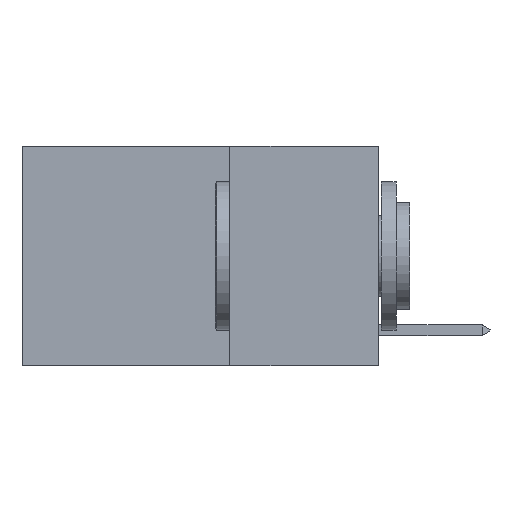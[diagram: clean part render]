
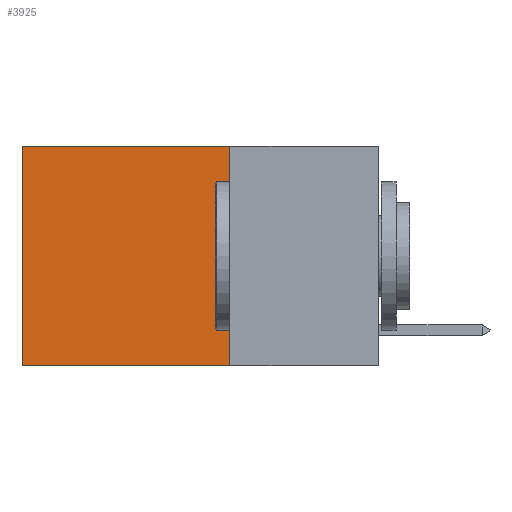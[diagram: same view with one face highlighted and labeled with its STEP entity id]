
A CAD part, left-side view. The second image highlights one B-rep face of the part: STEP entity #3925.
In plain terms, the highlighted planar face has unit normal (-1, 0, 0).
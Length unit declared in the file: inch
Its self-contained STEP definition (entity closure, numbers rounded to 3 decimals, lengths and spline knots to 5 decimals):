
#466 = CARTESIAN_POINT ( 'NONE',  ( 0.2625, 0.6, -0.37 ) ) ;
#601 = CARTESIAN_POINT ( 'NONE',  ( 0.2625, 0.25, 0. ) ) ;
#702 = DIRECTION ( 'NONE',  ( 0., 0., -1. ) ) ;
#2179 = DIRECTION ( 'NONE',  ( 0., 0., -1. ) ) ;
#2409 = CARTESIAN_POINT ( 'NONE',  ( 0.2625, 0.25, 0. ) ) ;
#3013 = LINE ( 'NONE', #16876, #23134 ) ;
#3422 = DIRECTION ( 'NONE',  ( 0., 1., 0. ) ) ;
#3453 = ORIENTED_EDGE ( 'NONE', *, *, #23475, .F. ) ;
#3925 = ADVANCED_FACE ( 'NONE', ( #22160 ), #12285, .F. ) ;
#4358 = CARTESIAN_POINT ( 'NONE',  ( 0.2625, 0.6, 0. ) ) ;
#4470 = DIRECTION ( 'NONE',  ( 0., 0., -1. ) ) ;
#4686 = ORIENTED_EDGE ( 'NONE', *, *, #4850, .T. ) ;
#4850 = EDGE_CURVE ( 'NONE', #19999, #11503, #18177, .T. ) ;
#4867 = CARTESIAN_POINT ( 'NONE',  ( 0.2625, 0.25, 0. ) ) ;
#6879 = DIRECTION ( 'NONE',  ( 0., 1., 0. ) ) ;
#7847 = VECTOR ( 'NONE', #6879, 39.37008 ) ;
#8093 = ORIENTED_EDGE ( 'NONE', *, *, #11638, .T. ) ;
#10164 = VECTOR ( 'NONE', #2179, 39.37008 ) ;
#10695 = VECTOR ( 'NONE', #702, 39.37008 ) ;
#11503 = VERTEX_POINT ( 'NONE', #13737 ) ;
#11638 = EDGE_CURVE ( 'NONE', #11503, #18515, #24910, .T. ) ;
#11917 = LINE ( 'NONE', #601, #10695 ) ;
#12285 = PLANE ( 'NONE',  #22256 ) ;
#13183 = VERTEX_POINT ( 'NONE', #22349 ) ;
#13350 = EDGE_CURVE ( 'NONE', #13183, #18515, #3013, .T. ) ;
#13737 = CARTESIAN_POINT ( 'NONE',  ( 0.2625, 0.6, 0. ) ) ;
#16202 = DIRECTION ( 'NONE',  ( 1., 0., 0. ) ) ;
#16876 = CARTESIAN_POINT ( 'NONE',  ( 0.2625, 0.25, -0.37 ) ) ;
#18177 = LINE ( 'NONE', #4867, #7847 ) ;
#18515 = VERTEX_POINT ( 'NONE', #466 ) ;
#19999 = VERTEX_POINT ( 'NONE', #20474 ) ;
#20474 = CARTESIAN_POINT ( 'NONE',  ( 0.2625, 0.25, 0. ) ) ;
#21687 = EDGE_LOOP ( 'NONE', ( #8093, #23517, #3453, #4686 ) ) ;
#22160 = FACE_OUTER_BOUND ( 'NONE', #21687, .T. ) ;
#22256 = AXIS2_PLACEMENT_3D ( 'NONE', #2409, #16202, #4470 ) ;
#22349 = CARTESIAN_POINT ( 'NONE',  ( 0.2625, 0.25, -0.37 ) ) ;
#23134 = VECTOR ( 'NONE', #3422, 39.37008 ) ;
#23475 = EDGE_CURVE ( 'NONE', #19999, #13183, #11917, .T. ) ;
#23517 = ORIENTED_EDGE ( 'NONE', *, *, #13350, .F. ) ;
#24910 = LINE ( 'NONE', #4358, #10164 ) ;
